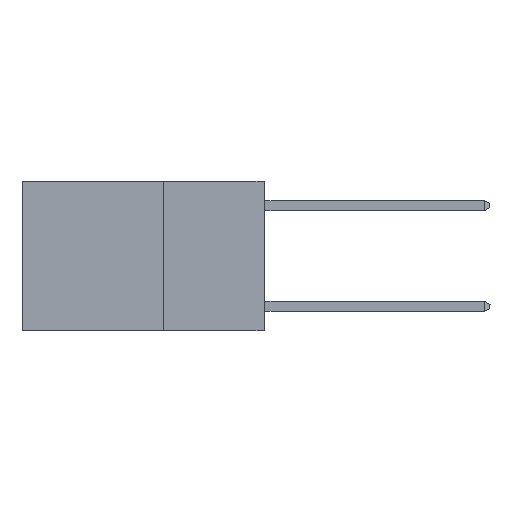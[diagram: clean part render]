
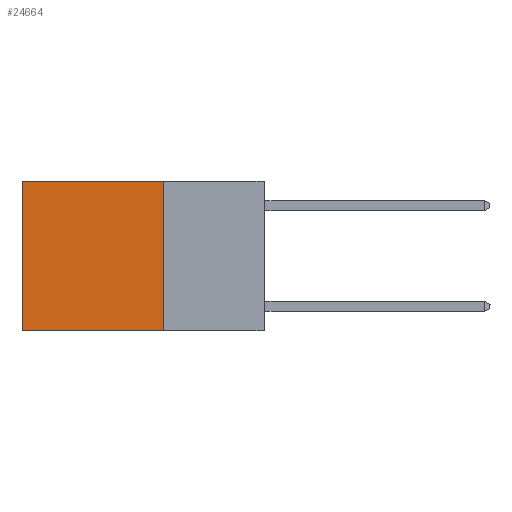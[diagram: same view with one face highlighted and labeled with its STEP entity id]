
A CAD part, left-side view. The second image highlights one B-rep face of the part: STEP entity #24664.
In plain terms, the highlighted planar face has unit normal (-1, 0, 0).
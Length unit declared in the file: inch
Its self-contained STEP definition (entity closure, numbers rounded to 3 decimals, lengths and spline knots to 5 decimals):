
#132 = DIRECTION ( 'NONE',  ( 0., 1., 0. ) ) ;
#408 = VERTEX_POINT ( 'NONE', #28128 ) ;
#518 = CARTESIAN_POINT ( 'NONE',  ( 0.2625, 0.6, 0. ) ) ;
#1718 = DIRECTION ( 'NONE',  ( 1., 0., 0. ) ) ;
#1725 = DIRECTION ( 'NONE',  ( 0., 0., -1. ) ) ;
#2485 = LINE ( 'NONE', #18678, #26972 ) ;
#3692 = EDGE_CURVE ( 'NONE', #408, #7245, #24016, .T. ) ;
#4752 = VERTEX_POINT ( 'NONE', #22948 ) ;
#5544 = CARTESIAN_POINT ( 'NONE',  ( 0.2625, 0.6, -0.37 ) ) ;
#7245 = VERTEX_POINT ( 'NONE', #7901 ) ;
#7296 = VERTEX_POINT ( 'NONE', #5544 ) ;
#7870 = DIRECTION ( 'NONE',  ( 0., 0., -1. ) ) ;
#7901 = CARTESIAN_POINT ( 'NONE',  ( 0.2625, 0.6, 0. ) ) ;
#8820 = EDGE_LOOP ( 'NONE', ( #9399, #18539, #17407, #14059 ) ) ;
#9399 = ORIENTED_EDGE ( 'NONE', *, *, #12367, .T. ) ;
#9968 = EDGE_CURVE ( 'NONE', #408, #4752, #2485, .T. ) ;
#11477 = EDGE_CURVE ( 'NONE', #4752, #7296, #24397, .T. ) ;
#12367 = EDGE_CURVE ( 'NONE', #7245, #7296, #14113, .T. ) ;
#12667 = VECTOR ( 'NONE', #23611, 39.37008 ) ;
#14059 = ORIENTED_EDGE ( 'NONE', *, *, #3692, .T. ) ;
#14113 = LINE ( 'NONE', #518, #19713 ) ;
#16630 = CARTESIAN_POINT ( 'NONE',  ( 0.2625, 0.25, -0.37 ) ) ;
#17407 = ORIENTED_EDGE ( 'NONE', *, *, #9968, .F. ) ;
#18539 = ORIENTED_EDGE ( 'NONE', *, *, #11477, .F. ) ;
#18672 = DIRECTION ( 'NONE',  ( 0., 0., -1. ) ) ;
#18678 = CARTESIAN_POINT ( 'NONE',  ( 0.2625, 0.25, 0. ) ) ;
#19396 = AXIS2_PLACEMENT_3D ( 'NONE', #29969, #1718, #18672 ) ;
#19713 = VECTOR ( 'NONE', #7870, 39.37008 ) ;
#22948 = CARTESIAN_POINT ( 'NONE',  ( 0.2625, 0.25, -0.37 ) ) ;
#23611 = DIRECTION ( 'NONE',  ( 0., 1., 0. ) ) ;
#24016 = LINE ( 'NONE', #26133, #29994 ) ;
#24255 = FACE_OUTER_BOUND ( 'NONE', #8820, .T. ) ;
#24397 = LINE ( 'NONE', #16630, #12667 ) ;
#24664 = ADVANCED_FACE ( 'NONE', ( #24255 ), #27696, .F. ) ;
#26133 = CARTESIAN_POINT ( 'NONE',  ( 0.2625, 0.25, 0. ) ) ;
#26972 = VECTOR ( 'NONE', #1725, 39.37008 ) ;
#27696 = PLANE ( 'NONE',  #19396 ) ;
#28128 = CARTESIAN_POINT ( 'NONE',  ( 0.2625, 0.25, 0. ) ) ;
#29969 = CARTESIAN_POINT ( 'NONE',  ( 0.2625, 0.25, 0. ) ) ;
#29994 = VECTOR ( 'NONE', #132, 39.37008 ) ;
